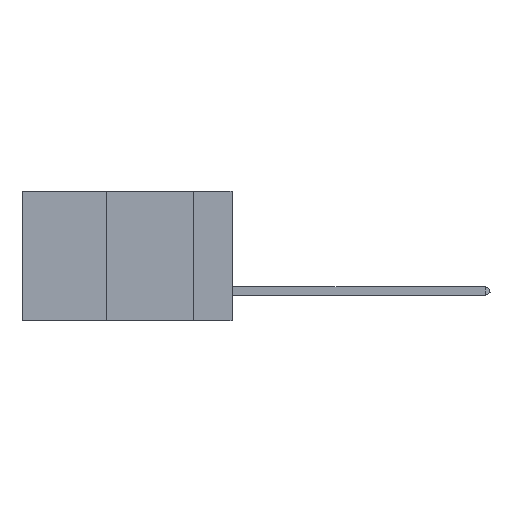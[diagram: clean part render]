
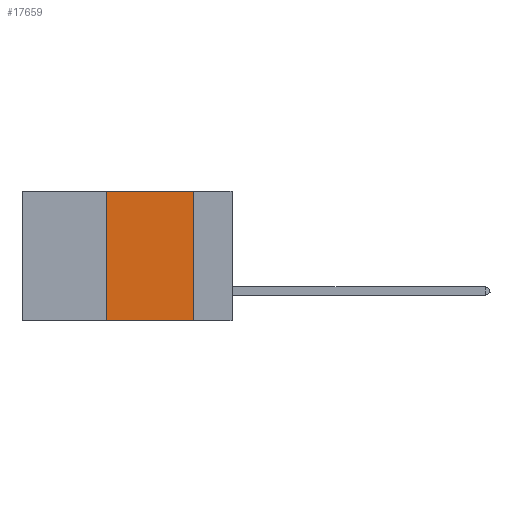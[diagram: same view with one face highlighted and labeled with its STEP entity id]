
A CAD part, left-side view. The second image highlights one B-rep face of the part: STEP entity #17659.
In plain terms, the highlighted planar face has unit normal (-1, 0, 0).
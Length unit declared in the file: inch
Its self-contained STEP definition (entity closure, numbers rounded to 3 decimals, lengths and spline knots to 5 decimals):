
#143 = CARTESIAN_POINT ( 'NONE',  ( 0., 0.11, 0. ) ) ;
#182 = AXIS2_PLACEMENT_3D ( 'NONE', #2199, #18545, #8049 ) ;
#506 = PLANE ( 'NONE',  #182 ) ;
#1392 = VECTOR ( 'NONE', #11554, 39.37008 ) ;
#1447 = EDGE_CURVE ( 'NONE', #11477, #16815, #16769, .T. ) ;
#2199 = CARTESIAN_POINT ( 'NONE',  ( 0., 0.6, 0. ) ) ;
#2453 = EDGE_CURVE ( 'NONE', #15641, #11477, #18620, .T. ) ;
#3267 = CARTESIAN_POINT ( 'NONE',  ( 0., 0.11, 0. ) ) ;
#3802 = VECTOR ( 'NONE', #17826, 39.37008 ) ;
#4189 = FACE_OUTER_BOUND ( 'NONE', #16543, .T. ) ;
#4875 = VECTOR ( 'NONE', #15507, 39.37008 ) ;
#5392 = EDGE_CURVE ( 'NONE', #15641, #16829, #22624, .T. ) ;
#6831 = EDGE_CURVE ( 'NONE', #16815, #16829, #10755, .T. ) ;
#6959 = DIRECTION ( 'NONE',  ( 0., -1., 0. ) ) ;
#8049 = DIRECTION ( 'NONE',  ( 0., 0., -1. ) ) ;
#10394 = CARTESIAN_POINT ( 'NONE',  ( 0., 0.36, -0.37 ) ) ;
#10755 = LINE ( 'NONE', #3267, #3802 ) ;
#10843 = CARTESIAN_POINT ( 'NONE',  ( 0., 0.36, 0. ) ) ;
#11394 = CARTESIAN_POINT ( 'NONE',  ( 0., 0.11, -0.37 ) ) ;
#11477 = VERTEX_POINT ( 'NONE', #10843 ) ;
#11522 = VECTOR ( 'NONE', #6959, 39.37008 ) ;
#11554 = DIRECTION ( 'NONE',  ( 0., -1., 0. ) ) ;
#11887 = ORIENTED_EDGE ( 'NONE', *, *, #5392, .T. ) ;
#11901 = CARTESIAN_POINT ( 'NONE',  ( 0., 0.36, 0. ) ) ;
#12597 = ORIENTED_EDGE ( 'NONE', *, *, #1447, .F. ) ;
#15507 = DIRECTION ( 'NONE',  ( 0., 0., 1. ) ) ;
#15641 = VERTEX_POINT ( 'NONE', #10394 ) ;
#15727 = CARTESIAN_POINT ( 'NONE',  ( 0., 0.6, 0. ) ) ;
#16543 = EDGE_LOOP ( 'NONE', ( #17511, #12597, #22430, #11887 ) ) ;
#16769 = LINE ( 'NONE', #15727, #11522 ) ;
#16815 = VERTEX_POINT ( 'NONE', #143 ) ;
#16829 = VERTEX_POINT ( 'NONE', #11394 ) ;
#17511 = ORIENTED_EDGE ( 'NONE', *, *, #6831, .F. ) ;
#17659 = ADVANCED_FACE ( 'NONE', ( #4189 ), #506, .F. ) ;
#17826 = DIRECTION ( 'NONE',  ( 0., 0., -1. ) ) ;
#18533 = CARTESIAN_POINT ( 'NONE',  ( 0., 0.6, -0.37 ) ) ;
#18545 = DIRECTION ( 'NONE',  ( 1., 0., 0. ) ) ;
#18620 = LINE ( 'NONE', #11901, #4875 ) ;
#22430 = ORIENTED_EDGE ( 'NONE', *, *, #2453, .F. ) ;
#22624 = LINE ( 'NONE', #18533, #1392 ) ;
